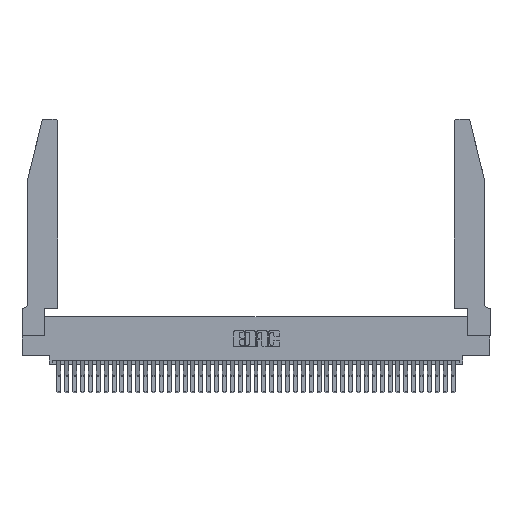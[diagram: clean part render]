
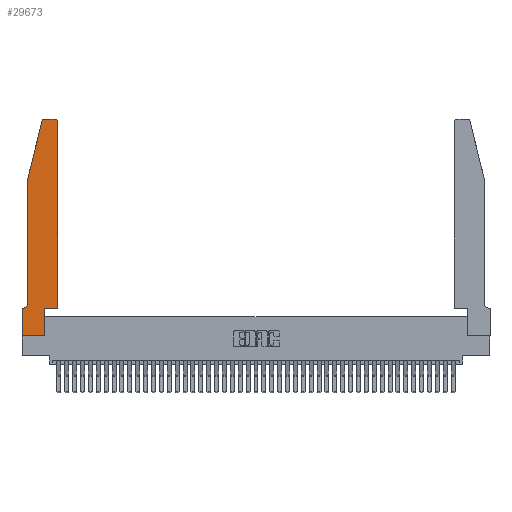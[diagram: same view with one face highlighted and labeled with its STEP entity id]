
A CAD part, top view. The second image highlights one B-rep face of the part: STEP entity #29673.
In plain terms, the highlighted planar face has unit normal (0, 0, 1).
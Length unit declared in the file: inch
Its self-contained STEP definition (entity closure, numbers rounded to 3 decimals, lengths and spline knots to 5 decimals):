
#99 = CARTESIAN_POINT ( 'NONE',  ( 0.4505, 2.72, 0.37 ) ) ;
#400 = VECTOR ( 'NONE', #11277, 39.37008 ) ;
#451 = AXIS2_PLACEMENT_3D ( 'NONE', #8440, #42051, #11730 ) ;
#1020 = DIRECTION ( 'NONE',  ( -1., 0., 0. ) ) ;
#1306 = CARTESIAN_POINT ( 'NONE',  ( 0.284, 2.72, 0.37 ) ) ;
#1461 = CARTESIAN_POINT ( 'NONE',  ( 0.4505, 0.35, 0.37 ) ) ;
#1932 = LINE ( 'NONE', #2150, #19407 ) ;
#2150 = CARTESIAN_POINT ( 'NONE',  ( 0.2605, 2.75, 0.37 ) ) ;
#2861 = LINE ( 'NONE', #12932, #33023 ) ;
#3399 = ORIENTED_EDGE ( 'NONE', *, *, #21425, .T. ) ;
#4507 = DIRECTION ( 'NONE',  ( 0., -1., 0. ) ) ;
#5439 = EDGE_CURVE ( 'NONE', #14296, #25493, #33227, .T. ) ;
#5959 = DIRECTION ( 'NONE',  ( 0., 1., 0. ) ) ;
#6017 = VERTEX_POINT ( 'NONE', #9366 ) ;
#6181 = LINE ( 'NONE', #34511, #7781 ) ;
#6719 = ORIENTED_EDGE ( 'NONE', *, *, #9275, .T. ) ;
#6958 = CARTESIAN_POINT ( 'NONE',  ( 0.2865, 0.35, 0.37 ) ) ;
#7146 = ORIENTED_EDGE ( 'NONE', *, *, #43617, .T. ) ;
#7187 = CARTESIAN_POINT ( 'NONE',  ( 0.4205, 2.72, 0.37 ) ) ;
#7311 = EDGE_CURVE ( 'NONE', #37455, #16663, #1932, .T. ) ;
#7781 = VECTOR ( 'NONE', #4507, 39.37008 ) ;
#8048 = VERTEX_POINT ( 'NONE', #41919 ) ;
#8440 = CARTESIAN_POINT ( 'NONE',  ( 0., 0.35, 0.37 ) ) ;
#9159 = ORIENTED_EDGE ( 'NONE', *, *, #14058, .T. ) ;
#9275 = EDGE_CURVE ( 'NONE', #40108, #10368, #22419, .T. ) ;
#9366 = CARTESIAN_POINT ( 'NONE',  ( 0.0755, 0.42, 0.37 ) ) ;
#9643 = VECTOR ( 'NONE', #1020, 39.37008 ) ;
#10053 = ORIENTED_EDGE ( 'NONE', *, *, #38642, .T. ) ;
#10294 = CIRCLE ( 'NONE', #26300, 0.03 ) ;
#10346 = CARTESIAN_POINT ( 'NONE',  ( 0.0055, 0.35, 0.37 ) ) ;
#10368 = VERTEX_POINT ( 'NONE', #11928 ) ;
#10910 = CIRCLE ( 'NONE', #38791, 0.03 ) ;
#11255 = ORIENTED_EDGE ( 'NONE', *, *, #7311, .T. ) ;
#11277 = DIRECTION ( 'NONE',  ( -0.239, -0.971, 0. ) ) ;
#11730 = DIRECTION ( 'NONE',  ( 1., 0., 0. ) ) ;
#11928 = CARTESIAN_POINT ( 'NONE',  ( 0., 0.35, 0.37 ) ) ;
#12250 = VERTEX_POINT ( 'NONE', #17487 ) ;
#12847 = EDGE_CURVE ( 'NONE', #30110, #12250, #19553, .T. ) ;
#12932 = CARTESIAN_POINT ( 'NONE',  ( 0., 0., 0.37 ) ) ;
#13558 = VECTOR ( 'NONE', #34959, 39.37008 ) ;
#14058 = EDGE_CURVE ( 'NONE', #6017, #40108, #21593, .T. ) ;
#14296 = VERTEX_POINT ( 'NONE', #22525 ) ;
#15719 = LINE ( 'NONE', #6958, #13558 ) ;
#16663 = VERTEX_POINT ( 'NONE', #25759 ) ;
#17329 = VECTOR ( 'NONE', #38299, 39.37008 ) ;
#17487 = CARTESIAN_POINT ( 'NONE',  ( 0.0755, 2., 0.37 ) ) ;
#17931 = ORIENTED_EDGE ( 'NONE', *, *, #27505, .T. ) ;
#18020 = VERTEX_POINT ( 'NONE', #23857 ) ;
#18079 = PLANE ( 'NONE',  #451 ) ;
#18499 = LINE ( 'NONE', #30080, #40674 ) ;
#19407 = VECTOR ( 'NONE', #21297, 39.37008 ) ;
#19553 = LINE ( 'NONE', #28166, #400 ) ;
#19905 = DIRECTION ( 'NONE',  ( 1., 0., 0. ) ) ;
#21297 = DIRECTION ( 'NONE',  ( -1., 0., 0. ) ) ;
#21425 = EDGE_CURVE ( 'NONE', #32513, #37455, #10294, .T. ) ;
#21593 = CIRCLE ( 'NONE', #35755, 0.07 ) ;
#22099 = ORIENTED_EDGE ( 'NONE', *, *, #12847, .T. ) ;
#22419 = LINE ( 'NONE', #35095, #9643 ) ;
#22424 = EDGE_CURVE ( 'NONE', #16663, #30110, #10910, .T. ) ;
#22525 = CARTESIAN_POINT ( 'NONE',  ( 0.2865, 0.35, 0.37 ) ) ;
#23837 = CARTESIAN_POINT ( 'NONE',  ( 0.25487, 2.72718, 0.37 ) ) ;
#23857 = CARTESIAN_POINT ( 'NONE',  ( 0.2865, 0., 0.37 ) ) ;
#24587 = DIRECTION ( 'NONE',  ( 1., 0., 0. ) ) ;
#24915 = VECTOR ( 'NONE', #5959, 39.37008 ) ;
#25045 = CARTESIAN_POINT ( 'NONE',  ( 0.4205, 2.75, 0.37 ) ) ;
#25493 = VERTEX_POINT ( 'NONE', #30825 ) ;
#25759 = CARTESIAN_POINT ( 'NONE',  ( 0.284, 2.75, 0.37 ) ) ;
#26182 = ORIENTED_EDGE ( 'NONE', *, *, #29393, .T. ) ;
#26300 = AXIS2_PLACEMENT_3D ( 'NONE', #7187, #37839, #24587 ) ;
#27360 = EDGE_CURVE ( 'NONE', #25493, #32513, #28619, .T. ) ;
#27505 = EDGE_CURVE ( 'NONE', #12250, #6017, #18499, .T. ) ;
#28166 = CARTESIAN_POINT ( 'NONE',  ( 0.0755, 2., 0.37 ) ) ;
#28619 = LINE ( 'NONE', #31251, #24915 ) ;
#29201 = ORIENTED_EDGE ( 'NONE', *, *, #22424, .T. ) ;
#29383 = DIRECTION ( 'NONE',  ( 0., 0., -1. ) ) ;
#29393 = EDGE_CURVE ( 'NONE', #8048, #18020, #2861, .T. ) ;
#29673 = ADVANCED_FACE ( 'NONE', ( #40918 ), #18079, .T. ) ;
#30080 = CARTESIAN_POINT ( 'NONE',  ( 0.0755, 2., 0.37 ) ) ;
#30110 = VERTEX_POINT ( 'NONE', #23837 ) ;
#30825 = CARTESIAN_POINT ( 'NONE',  ( 0.4505, 0.35, 0.37 ) ) ;
#31251 = CARTESIAN_POINT ( 'NONE',  ( 0.4505, 0.35, 0.37 ) ) ;
#32513 = VERTEX_POINT ( 'NONE', #99 ) ;
#32613 = CARTESIAN_POINT ( 'NONE',  ( 0.0055, 0.42, 0.37 ) ) ;
#32700 = ORIENTED_EDGE ( 'NONE', *, *, #27360, .T. ) ;
#33023 = VECTOR ( 'NONE', #19905, 39.37008 ) ;
#33227 = LINE ( 'NONE', #1461, #17329 ) ;
#34511 = CARTESIAN_POINT ( 'NONE',  ( 0., 0., 0.37 ) ) ;
#34959 = DIRECTION ( 'NONE',  ( 0., 1., 0. ) ) ;
#35095 = CARTESIAN_POINT ( 'NONE',  ( 0.0755, 0.35, 0.37 ) ) ;
#35755 = AXIS2_PLACEMENT_3D ( 'NONE', #32613, #29383, #43396 ) ;
#35957 = DIRECTION ( 'NONE',  ( 0., 0., 1. ) ) ;
#37455 = VERTEX_POINT ( 'NONE', #25045 ) ;
#37839 = DIRECTION ( 'NONE',  ( 0., 0., 1. ) ) ;
#38299 = DIRECTION ( 'NONE',  ( 1., 0., 0. ) ) ;
#38642 = EDGE_CURVE ( 'NONE', #18020, #14296, #15719, .T. ) ;
#38791 = AXIS2_PLACEMENT_3D ( 'NONE', #1306, #35957, #39507 ) ;
#39507 = DIRECTION ( 'NONE',  ( 1., 0., 0. ) ) ;
#40108 = VERTEX_POINT ( 'NONE', #10346 ) ;
#40261 = DIRECTION ( 'NONE',  ( 0., -1., 0. ) ) ;
#40674 = VECTOR ( 'NONE', #40261, 39.37008 ) ;
#40918 = FACE_OUTER_BOUND ( 'NONE', #41659, .T. ) ;
#41489 = ORIENTED_EDGE ( 'NONE', *, *, #5439, .T. ) ;
#41659 = EDGE_LOOP ( 'NONE', ( #11255, #29201, #22099, #17931, #9159, #6719, #7146, #26182, #10053, #41489, #32700, #3399 ) ) ;
#41919 = CARTESIAN_POINT ( 'NONE',  ( 0., 0., 0.37 ) ) ;
#42051 = DIRECTION ( 'NONE',  ( 0., 0., 1. ) ) ;
#43396 = DIRECTION ( 'NONE',  ( -1., 0., 0. ) ) ;
#43617 = EDGE_CURVE ( 'NONE', #10368, #8048, #6181, .T. ) ;
